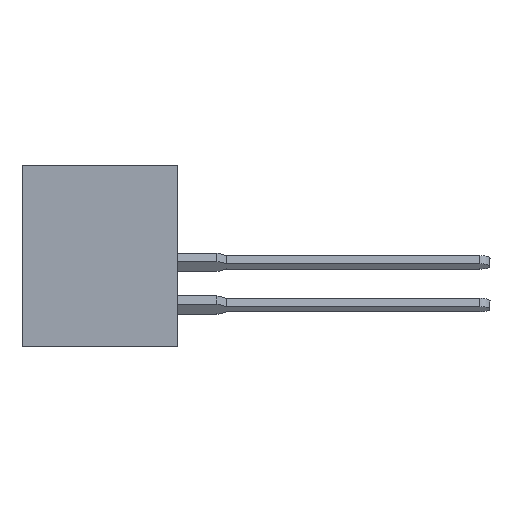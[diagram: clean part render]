
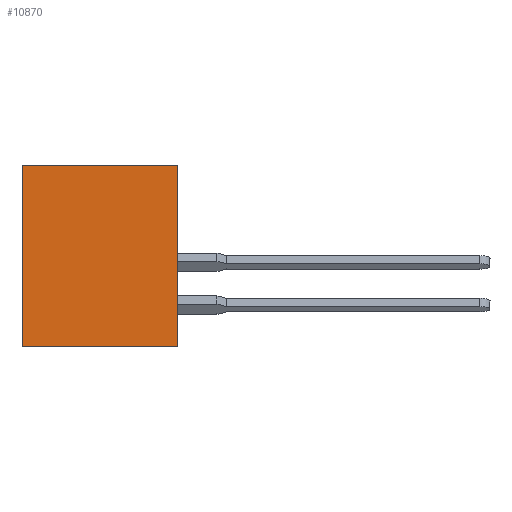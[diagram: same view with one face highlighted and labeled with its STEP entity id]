
A CAD part, left-side view. The second image highlights one B-rep face of the part: STEP entity #10870.
In plain terms, the highlighted planar face has unit normal (-1, 0, 0).
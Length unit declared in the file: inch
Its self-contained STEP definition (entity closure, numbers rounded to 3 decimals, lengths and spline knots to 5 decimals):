
#165 = FACE_OUTER_BOUND ( 'NONE', #16893, .T. ) ;
#1309 = EDGE_CURVE ( 'NONE', #9625, #9304, #2032, .T. ) ;
#1598 = CARTESIAN_POINT ( 'NONE',  ( 0., 0.453, 0. ) ) ;
#2032 = LINE ( 'NONE', #14745, #13055 ) ;
#2164 = LINE ( 'NONE', #8202, #11103 ) ;
#2444 = ORIENTED_EDGE ( 'NONE', *, *, #14727, .F. ) ;
#3037 = EDGE_CURVE ( 'NONE', #9304, #13203, #12534, .T. ) ;
#4281 = DIRECTION ( 'NONE',  ( 1., 0., 0. ) ) ;
#4961 = ORIENTED_EDGE ( 'NONE', *, *, #3037, .T. ) ;
#5834 = DIRECTION ( 'NONE',  ( 0., -1., 0. ) ) ;
#8202 = CARTESIAN_POINT ( 'NONE',  ( 0., 0.453, 0. ) ) ;
#8979 = DIRECTION ( 'NONE',  ( 0., -1., 0. ) ) ;
#9304 = VERTEX_POINT ( 'NONE', #17570 ) ;
#9625 = VERTEX_POINT ( 'NONE', #14522 ) ;
#9904 = ORIENTED_EDGE ( 'NONE', *, *, #13475, .F. ) ;
#10090 = LINE ( 'NONE', #1598, #10795 ) ;
#10423 = VERTEX_POINT ( 'NONE', #16977 ) ;
#10795 = VECTOR ( 'NONE', #8979, 39.37008 ) ;
#10870 = ADVANCED_FACE ( 'NONE', ( #165 ), #17723, .F. ) ;
#11103 = VECTOR ( 'NONE', #14185, 39.37008 ) ;
#11875 = CARTESIAN_POINT ( 'NONE',  ( 0., 0., 0. ) ) ;
#12534 = LINE ( 'NONE', #11875, #15550 ) ;
#13055 = VECTOR ( 'NONE', #5834, 39.37008 ) ;
#13203 = VERTEX_POINT ( 'NONE', #18996 ) ;
#13475 = EDGE_CURVE ( 'NONE', #9625, #10423, #2164, .T. ) ;
#14185 = DIRECTION ( 'NONE',  ( 0., 0., 1. ) ) ;
#14522 = CARTESIAN_POINT ( 'NONE',  ( 0., 0.453, -0.531 ) ) ;
#14727 = EDGE_CURVE ( 'NONE', #10423, #13203, #10090, .T. ) ;
#14745 = CARTESIAN_POINT ( 'NONE',  ( 0., 0.453, -0.531 ) ) ;
#15550 = VECTOR ( 'NONE', #16266, 39.37008 ) ;
#16218 = CARTESIAN_POINT ( 'NONE',  ( 0., 0.453, 0. ) ) ;
#16266 = DIRECTION ( 'NONE',  ( 0., 0., 1. ) ) ;
#16784 = AXIS2_PLACEMENT_3D ( 'NONE', #16218, #4281, #17102 ) ;
#16893 = EDGE_LOOP ( 'NONE', ( #4961, #2444, #9904, #16995 ) ) ;
#16977 = CARTESIAN_POINT ( 'NONE',  ( 0., 0.453, 0. ) ) ;
#16995 = ORIENTED_EDGE ( 'NONE', *, *, #1309, .T. ) ;
#17102 = DIRECTION ( 'NONE',  ( 0., 0., -1. ) ) ;
#17570 = CARTESIAN_POINT ( 'NONE',  ( 0., 0., -0.531 ) ) ;
#17723 = PLANE ( 'NONE',  #16784 ) ;
#18996 = CARTESIAN_POINT ( 'NONE',  ( 0., 0., 0. ) ) ;
